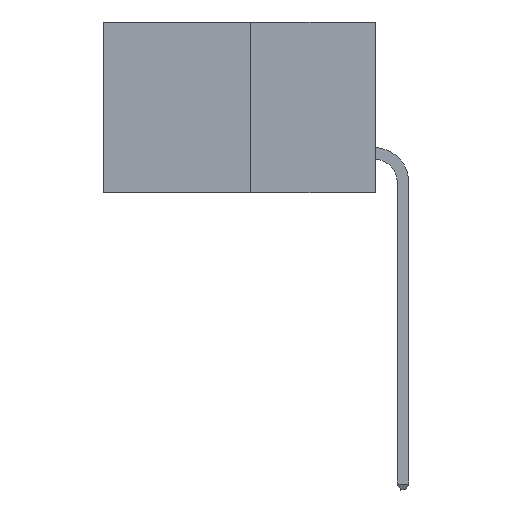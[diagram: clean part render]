
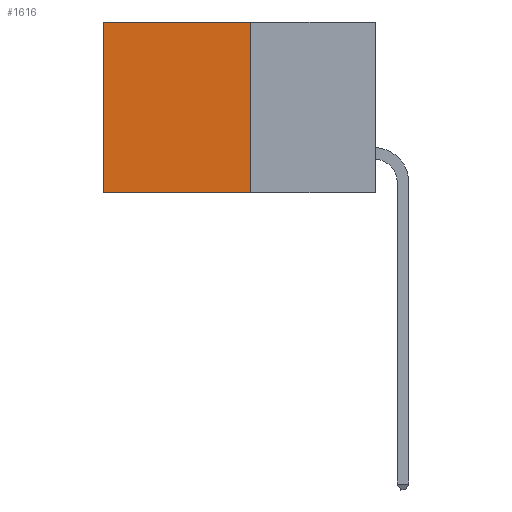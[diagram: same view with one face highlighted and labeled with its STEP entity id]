
A CAD part, left-side view. The second image highlights one B-rep face of the part: STEP entity #1616.
In plain terms, the highlighted planar face has unit normal (-1, 0, 0).
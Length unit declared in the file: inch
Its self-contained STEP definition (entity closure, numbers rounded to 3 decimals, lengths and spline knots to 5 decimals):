
#309 = CARTESIAN_POINT ( 'NONE',  ( 0.277, 0.27, 0. ) ) ;
#830 = VECTOR ( 'NONE', #3637, 39.37008 ) ;
#1211 = DIRECTION ( 'NONE',  ( 0., 1., 0. ) ) ;
#1250 = CARTESIAN_POINT ( 'NONE',  ( 0.277, 0.27, -0.37 ) ) ;
#1426 = LINE ( 'NONE', #5891, #3474 ) ;
#1494 = ORIENTED_EDGE ( 'NONE', *, *, #5232, .F. ) ;
#1616 = ADVANCED_FACE ( 'NONE', ( #7222 ), #6443, .F. ) ;
#1975 = CARTESIAN_POINT ( 'NONE',  ( 0.277, 0.27, -0.37 ) ) ;
#2584 = VERTEX_POINT ( 'NONE', #6714 ) ;
#2996 = CARTESIAN_POINT ( 'NONE',  ( 0.277, 0.59, 0. ) ) ;
#3474 = VECTOR ( 'NONE', #6764, 39.37008 ) ;
#3483 = ORIENTED_EDGE ( 'NONE', *, *, #7945, .T. ) ;
#3637 = DIRECTION ( 'NONE',  ( 0., 1., 0. ) ) ;
#3725 = CARTESIAN_POINT ( 'NONE',  ( 0.277, 0.59, -0.37 ) ) ;
#3884 = VECTOR ( 'NONE', #6957, 39.37008 ) ;
#4343 = EDGE_CURVE ( 'NONE', #9204, #2584, #10820, .T. ) ;
#5232 = EDGE_CURVE ( 'NONE', #2584, #6950, #11008, .T. ) ;
#5891 = CARTESIAN_POINT ( 'NONE',  ( 0.277, 0.59, -0.37 ) ) ;
#6443 = PLANE ( 'NONE',  #10400 ) ;
#6714 = CARTESIAN_POINT ( 'NONE',  ( 0.277, 0.27, -0.37 ) ) ;
#6764 = DIRECTION ( 'NONE',  ( 0., 0., -1. ) ) ;
#6950 = VERTEX_POINT ( 'NONE', #3725 ) ;
#6957 = DIRECTION ( 'NONE',  ( 0., 0., -1. ) ) ;
#6996 = CARTESIAN_POINT ( 'NONE',  ( 0.277, 0.27, -0.37 ) ) ;
#7222 = FACE_OUTER_BOUND ( 'NONE', #11123, .T. ) ;
#7715 = VERTEX_POINT ( 'NONE', #2996 ) ;
#7945 = EDGE_CURVE ( 'NONE', #7715, #6950, #1426, .T. ) ;
#8033 = CARTESIAN_POINT ( 'NONE',  ( 0.277, 0.27, 0. ) ) ;
#8481 = VECTOR ( 'NONE', #1211, 39.37008 ) ;
#9159 = ORIENTED_EDGE ( 'NONE', *, *, #4343, .F. ) ;
#9204 = VERTEX_POINT ( 'NONE', #309 ) ;
#9514 = ORIENTED_EDGE ( 'NONE', *, *, #9911, .T. ) ;
#9518 = DIRECTION ( 'NONE',  ( 1., 0., 0. ) ) ;
#9842 = LINE ( 'NONE', #8033, #830 ) ;
#9911 = EDGE_CURVE ( 'NONE', #9204, #7715, #9842, .T. ) ;
#9918 = DIRECTION ( 'NONE',  ( 0., 0., -1. ) ) ;
#10400 = AXIS2_PLACEMENT_3D ( 'NONE', #1975, #9518, #9918 ) ;
#10820 = LINE ( 'NONE', #6996, #3884 ) ;
#11008 = LINE ( 'NONE', #1250, #8481 ) ;
#11123 = EDGE_LOOP ( 'NONE', ( #3483, #1494, #9159, #9514 ) ) ;
